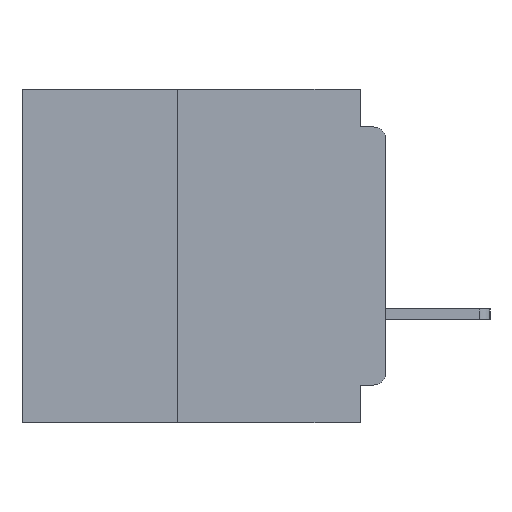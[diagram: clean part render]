
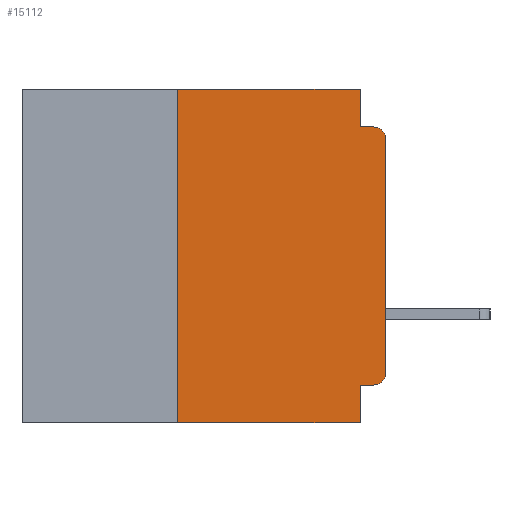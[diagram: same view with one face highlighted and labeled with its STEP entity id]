
A CAD part, left-side view. The second image highlights one B-rep face of the part: STEP entity #15112.
In plain terms, the highlighted planar face has unit normal (-1, 0, 0).
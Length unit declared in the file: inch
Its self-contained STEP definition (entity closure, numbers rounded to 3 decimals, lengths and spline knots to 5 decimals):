
#2230 = LINE ( 'NONE', #4273, #36018 ) ;
#2531 = VECTOR ( 'NONE', #29390, 39.37008 ) ;
#2672 = EDGE_CURVE ( 'NONE', #37420, #25013, #31735, .T. ) ;
#2717 = DIRECTION ( 'NONE',  ( 0., -1., 0. ) ) ;
#3462 = EDGE_CURVE ( 'NONE', #28012, #27729, #35738, .T. ) ;
#4033 = PLANE ( 'NONE',  #17065 ) ;
#4178 = CARTESIAN_POINT ( 'NONE',  ( 0., 0.015, -0.045 ) ) ;
#4273 = CARTESIAN_POINT ( 'NONE',  ( 0., 0.437, -0.4 ) ) ;
#4281 = ORIENTED_EDGE ( 'NONE', *, *, #37902, .F. ) ;
#4727 = CARTESIAN_POINT ( 'NONE',  ( 0., 0.015, -0.06 ) ) ;
#4942 = CARTESIAN_POINT ( 'NONE',  ( 0., 0.031, -0.4 ) ) ;
#5664 = CARTESIAN_POINT ( 'NONE',  ( 0., 0.25, -0.4 ) ) ;
#6168 = ORIENTED_EDGE ( 'NONE', *, *, #23286, .F. ) ;
#6611 = DIRECTION ( 'NONE',  ( -1., 0., 0. ) ) ;
#6883 = EDGE_CURVE ( 'NONE', #17668, #41767, #39482, .T. ) ;
#8017 = DIRECTION ( 'NONE',  ( 0., 0., -1. ) ) ;
#8167 = VECTOR ( 'NONE', #14619, 39.37008 ) ;
#8204 = VERTEX_POINT ( 'NONE', #4942 ) ;
#8347 = VERTEX_POINT ( 'NONE', #5664 ) ;
#8774 = CARTESIAN_POINT ( 'NONE',  ( 0., 0., -0.06 ) ) ;
#9048 = EDGE_CURVE ( 'NONE', #30625, #32936, #12418, .T. ) ;
#9061 = ORIENTED_EDGE ( 'NONE', *, *, #25734, .T. ) ;
#9304 = CARTESIAN_POINT ( 'NONE',  ( 0., 0.437, 0. ) ) ;
#9939 = CARTESIAN_POINT ( 'NONE',  ( 0., 0., -0.045 ) ) ;
#10294 = EDGE_CURVE ( 'NONE', #32936, #17668, #28655, .T. ) ;
#10980 = DIRECTION ( 'NONE',  ( 0., -1., 0. ) ) ;
#11341 = CARTESIAN_POINT ( 'NONE',  ( 0., 0.031, -0.4 ) ) ;
#11364 = VECTOR ( 'NONE', #2717, 39.37008 ) ;
#12343 = AXIS2_PLACEMENT_3D ( 'NONE', #26199, #6611, #29467 ) ;
#12418 = LINE ( 'NONE', #9304, #11364 ) ;
#12899 = ORIENTED_EDGE ( 'NONE', *, *, #2672, .T. ) ;
#12979 = ORIENTED_EDGE ( 'NONE', *, *, #31285, .T. ) ;
#14352 = ORIENTED_EDGE ( 'NONE', *, *, #6883, .F. ) ;
#14619 = DIRECTION ( 'NONE',  ( 0., 0., -1. ) ) ;
#15112 = ADVANCED_FACE ( 'NONE', ( #36634 ), #4033, .F. ) ;
#15405 = CARTESIAN_POINT ( 'NONE',  ( 0., 0.031, -0.355 ) ) ;
#15908 = DIRECTION ( 'NONE',  ( 0., 0., 1. ) ) ;
#16880 = LINE ( 'NONE', #11341, #8167 ) ;
#17065 = AXIS2_PLACEMENT_3D ( 'NONE', #36749, #39992, #20506 ) ;
#17290 = DIRECTION ( 'NONE',  ( 0., 1., 0. ) ) ;
#17668 = VERTEX_POINT ( 'NONE', #30851 ) ;
#18403 = VECTOR ( 'NONE', #17290, 39.37008 ) ;
#19861 = DIRECTION ( 'NONE',  ( 0., -1., 0. ) ) ;
#20506 = DIRECTION ( 'NONE',  ( 0., 0., -1. ) ) ;
#20810 = CARTESIAN_POINT ( 'NONE',  ( 0., 0.25, 0. ) ) ;
#21578 = ORIENTED_EDGE ( 'NONE', *, *, #22552, .T. ) ;
#22000 = VECTOR ( 'NONE', #15908, 39.37008 ) ;
#22083 = DIRECTION ( 'NONE',  ( 0., 0., 1. ) ) ;
#22137 = VECTOR ( 'NONE', #19861, 39.37008 ) ;
#22552 = EDGE_CURVE ( 'NONE', #8347, #8204, #2230, .T. ) ;
#23286 = EDGE_CURVE ( 'NONE', #8347, #30625, #34406, .T. ) ;
#23734 = CARTESIAN_POINT ( 'NONE',  ( 0., 0., -0.355 ) ) ;
#24069 = CIRCLE ( 'NONE', #36877, 0.015 ) ;
#25013 = VERTEX_POINT ( 'NONE', #8774 ) ;
#25646 = CARTESIAN_POINT ( 'NONE',  ( 0., 0., 0. ) ) ;
#25734 = EDGE_CURVE ( 'NONE', #28012, #37420, #38738, .T. ) ;
#26199 = CARTESIAN_POINT ( 'NONE',  ( 0., 0.015, -0.34 ) ) ;
#27597 = DIRECTION ( 'NONE',  ( -1., 0., 0. ) ) ;
#27729 = VERTEX_POINT ( 'NONE', #15405 ) ;
#28012 = VERTEX_POINT ( 'NONE', #36525 ) ;
#28655 = LINE ( 'NONE', #32664, #2531 ) ;
#29390 = DIRECTION ( 'NONE',  ( 0., 0., -1. ) ) ;
#29467 = DIRECTION ( 'NONE',  ( 0., 0., -1. ) ) ;
#29700 = ORIENTED_EDGE ( 'NONE', *, *, #9048, .F. ) ;
#30625 = VERTEX_POINT ( 'NONE', #20810 ) ;
#30851 = CARTESIAN_POINT ( 'NONE',  ( 0., 0.031, -0.045 ) ) ;
#31285 = EDGE_CURVE ( 'NONE', #25013, #41767, #24069, .T. ) ;
#31735 = LINE ( 'NONE', #25646, #22000 ) ;
#32108 = ORIENTED_EDGE ( 'NONE', *, *, #3462, .F. ) ;
#32664 = CARTESIAN_POINT ( 'NONE',  ( 0., 0.031, 0. ) ) ;
#32936 = VERTEX_POINT ( 'NONE', #39707 ) ;
#33030 = EDGE_LOOP ( 'NONE', ( #12899, #12979, #14352, #38759, #29700, #6168, #21578, #4281, #32108, #9061 ) ) ;
#34406 = LINE ( 'NONE', #41558, #35450 ) ;
#35450 = VECTOR ( 'NONE', #22083, 39.37008 ) ;
#35738 = LINE ( 'NONE', #23734, #18403 ) ;
#36018 = VECTOR ( 'NONE', #10980, 39.37008 ) ;
#36525 = CARTESIAN_POINT ( 'NONE',  ( 0., 0.015, -0.355 ) ) ;
#36634 = FACE_OUTER_BOUND ( 'NONE', #33030, .T. ) ;
#36749 = CARTESIAN_POINT ( 'NONE',  ( 0., 0.437, 0. ) ) ;
#36877 = AXIS2_PLACEMENT_3D ( 'NONE', #4727, #27597, #8017 ) ;
#37420 = VERTEX_POINT ( 'NONE', #41443 ) ;
#37902 = EDGE_CURVE ( 'NONE', #27729, #8204, #16880, .T. ) ;
#38738 = CIRCLE ( 'NONE', #12343, 0.015 ) ;
#38759 = ORIENTED_EDGE ( 'NONE', *, *, #10294, .F. ) ;
#39482 = LINE ( 'NONE', #9939, #22137 ) ;
#39707 = CARTESIAN_POINT ( 'NONE',  ( 0., 0.031, 0. ) ) ;
#39992 = DIRECTION ( 'NONE',  ( 1., 0., 0. ) ) ;
#41443 = CARTESIAN_POINT ( 'NONE',  ( 0., 0., -0.34 ) ) ;
#41558 = CARTESIAN_POINT ( 'NONE',  ( 0., 0.25, -0.4 ) ) ;
#41767 = VERTEX_POINT ( 'NONE', #4178 ) ;
